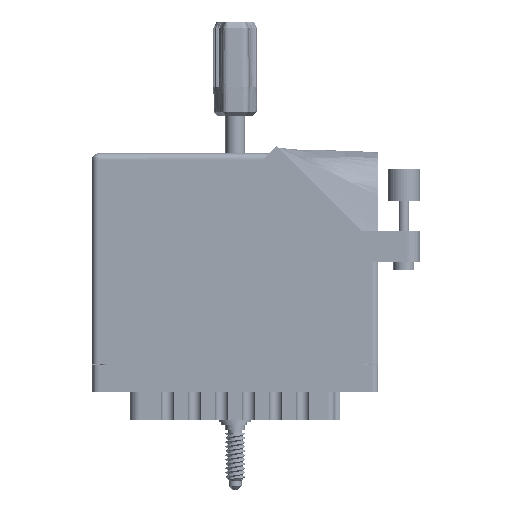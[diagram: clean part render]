
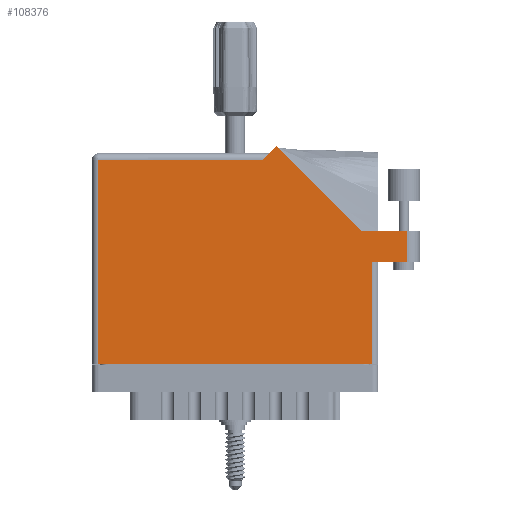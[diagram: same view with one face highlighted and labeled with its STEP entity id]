
A CAD part, front view. The second image highlights one B-rep face of the part: STEP entity #108376.
In plain terms, the highlighted face is planar.
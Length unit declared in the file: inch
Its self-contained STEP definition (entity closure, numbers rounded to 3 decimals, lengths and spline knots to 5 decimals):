
#1821 = ORIENTED_EDGE ( 'NONE', *, *, #33239, .T. ) ;
#8776 = VERTEX_POINT ( 'NONE', #80808 ) ;
#10046 = VECTOR ( 'NONE', #49509, 39.37008 ) ;
#10085 = EDGE_CURVE ( 'NONE', #8776, #98786, #60117, .T. ) ;
#11933 = LINE ( 'NONE', #28630, #97922 ) ;
#12442 = CARTESIAN_POINT ( 'NONE',  ( 0., 2.03, 0. ) ) ;
#13155 = ORIENTED_EDGE ( 'NONE', *, *, #69923, .T. ) ;
#13542 = PLANE ( 'NONE',  #26849 ) ;
#13651 = LINE ( 'NONE', #18216, #25503 ) ;
#14186 = CARTESIAN_POINT ( 'NONE',  ( 0.062, 1.968, 0. ) ) ;
#16565 = EDGE_CURVE ( 'NONE', #48117, #67699, #65554, .T. ) ;
#17778 = DIRECTION ( 'NONE',  ( -1., 0., 0. ) ) ;
#18216 = CARTESIAN_POINT ( 'NONE',  ( 3.03, 1.287, 0. ) ) ;
#19845 = EDGE_CURVE ( 'NONE', #47788, #48117, #11933, .T. ) ;
#20260 = ORIENTED_EDGE ( 'NONE', *, *, #19845, .T. ) ;
#20602 = CARTESIAN_POINT ( 'NONE',  ( 2.693, 0.98, 0. ) ) ;
#20985 = DIRECTION ( 'NONE',  ( 0., 1., 0. ) ) ;
#21301 = DIRECTION ( 'NONE',  ( 0., 0., -1. ) ) ;
#25503 = VECTOR ( 'NONE', #60372, 39.37008 ) ;
#26849 = AXIS2_PLACEMENT_3D ( 'NONE', #12442, #21301, #30176 ) ;
#26903 = VECTOR ( 'NONE', #76911, 39.37008 ) ;
#28630 = CARTESIAN_POINT ( 'NONE',  ( 0.062, 0., 0. ) ) ;
#30154 = CARTESIAN_POINT ( 'NONE',  ( 1.643, 1.968, 0. ) ) ;
#30176 = DIRECTION ( 'NONE',  ( -1., 0., 0. ) ) ;
#32577 = LINE ( 'NONE', #50939, #10046 ) ;
#33239 = EDGE_CURVE ( 'NONE', #36576, #8776, #46629, .T. ) ;
#36576 = VERTEX_POINT ( 'NONE', #74173 ) ;
#38352 = EDGE_CURVE ( 'NONE', #67699, #101816, #84135, .T. ) ;
#38664 = LINE ( 'NONE', #51051, #55821 ) ;
#39101 = VECTOR ( 'NONE', #64945, 39.37008 ) ;
#43371 = CARTESIAN_POINT ( 'NONE',  ( 3.03, 1.287, 0. ) ) ;
#43644 = CARTESIAN_POINT ( 'NONE',  ( 0.062, 0., 0. ) ) ;
#44551 = ORIENTED_EDGE ( 'NONE', *, *, #16565, .T. ) ;
#45378 = CARTESIAN_POINT ( 'NONE',  ( 2.755, 0.98, 0. ) ) ;
#45745 = LINE ( 'NONE', #45378, #66930 ) ;
#46529 = ORIENTED_EDGE ( 'NONE', *, *, #38352, .T. ) ;
#46629 = LINE ( 'NONE', #68580, #58535 ) ;
#47163 = ORIENTED_EDGE ( 'NONE', *, *, #75592, .T. ) ;
#47788 = VERTEX_POINT ( 'NONE', #14186 ) ;
#48117 = VERTEX_POINT ( 'NONE', #43644 ) ;
#49509 = DIRECTION ( 'NONE',  ( -1., 0., 0. ) ) ;
#50939 = CARTESIAN_POINT ( 'NONE',  ( 3.155, 1.287, 0. ) ) ;
#51051 = CARTESIAN_POINT ( 'NONE',  ( 0., 1.968, 0. ) ) ;
#52095 = CARTESIAN_POINT ( 'NONE',  ( 1.705, 2.03, 0. ) ) ;
#52413 = CARTESIAN_POINT ( 'NONE',  ( 2.693, 0.98, 0. ) ) ;
#55184 = VECTOR ( 'NONE', #20985, 39.37008 ) ;
#55821 = VECTOR ( 'NONE', #17778, 39.37008 ) ;
#58535 = VECTOR ( 'NONE', #70019, 39.37008 ) ;
#59798 = VERTEX_POINT ( 'NONE', #66973 ) ;
#60117 = LINE ( 'NONE', #52095, #26903 ) ;
#60372 = DIRECTION ( 'NONE',  ( 0., 1., 0. ) ) ;
#62037 = DIRECTION ( 'NONE',  ( 1., 0., 0. ) ) ;
#64148 = EDGE_CURVE ( 'NONE', #68497, #36576, #32577, .T. ) ;
#64945 = DIRECTION ( 'NONE',  ( 1., 0., 0. ) ) ;
#65554 = LINE ( 'NONE', #99258, #39101 ) ;
#66930 = VECTOR ( 'NONE', #62037, 39.37008 ) ;
#66973 = CARTESIAN_POINT ( 'NONE',  ( 3.03, 0.98, 0. ) ) ;
#67699 = VERTEX_POINT ( 'NONE', #108259 ) ;
#68497 = VERTEX_POINT ( 'NONE', #43371 ) ;
#68580 = CARTESIAN_POINT ( 'NONE',  ( 2.58942, 1.287, 0. ) ) ;
#69923 = EDGE_CURVE ( 'NONE', #98786, #47788, #38664, .T. ) ;
#70019 = DIRECTION ( 'NONE',  ( -0.707, 0.707, 0. ) ) ;
#73616 = EDGE_CURVE ( 'NONE', #101816, #59798, #45745, .T. ) ;
#74173 = CARTESIAN_POINT ( 'NONE',  ( 2.58942, 1.287, 0. ) ) ;
#75592 = EDGE_CURVE ( 'NONE', #59798, #68497, #13651, .T. ) ;
#76911 = DIRECTION ( 'NONE',  ( -0.707, -0.707, 0. ) ) ;
#80808 = CARTESIAN_POINT ( 'NONE',  ( 1.77571, 2.10071, 0. ) ) ;
#84135 = LINE ( 'NONE', #20602, #55184 ) ;
#84433 = ORIENTED_EDGE ( 'NONE', *, *, #73616, .T. ) ;
#87326 = ORIENTED_EDGE ( 'NONE', *, *, #10085, .T. ) ;
#87782 = DIRECTION ( 'NONE',  ( 0., -1., 0. ) ) ;
#94389 = FACE_OUTER_BOUND ( 'NONE', #107689, .T. ) ;
#97922 = VECTOR ( 'NONE', #87782, 39.37008 ) ;
#98786 = VERTEX_POINT ( 'NONE', #30154 ) ;
#99258 = CARTESIAN_POINT ( 'NONE',  ( 0., 0., 0. ) ) ;
#101640 = ORIENTED_EDGE ( 'NONE', *, *, #64148, .T. ) ;
#101816 = VERTEX_POINT ( 'NONE', #52413 ) ;
#107689 = EDGE_LOOP ( 'NONE', ( #84433, #47163, #101640, #1821, #87326, #13155, #20260, #44551, #46529 ) ) ;
#108259 = CARTESIAN_POINT ( 'NONE',  ( 2.693, 0., 0. ) ) ;
#108376 = ADVANCED_FACE ( 'NONE', ( #94389 ), #13542, .F. ) ;
